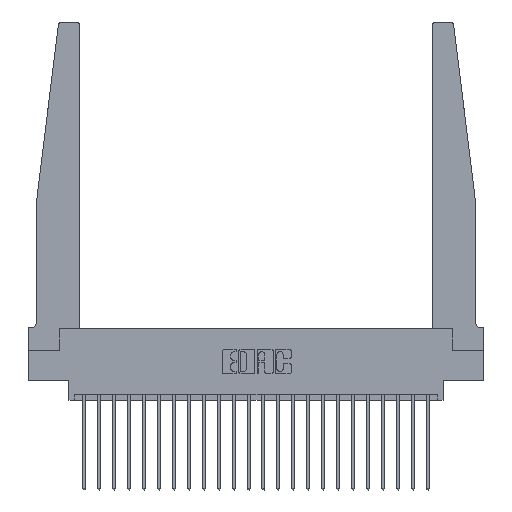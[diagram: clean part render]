
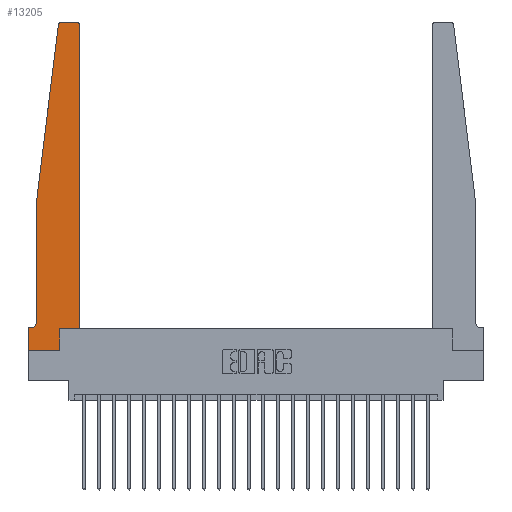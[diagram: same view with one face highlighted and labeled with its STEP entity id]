
A CAD part, top view. The second image highlights one B-rep face of the part: STEP entity #13205.
In plain terms, the highlighted planar face has unit normal (0, 0, 1).
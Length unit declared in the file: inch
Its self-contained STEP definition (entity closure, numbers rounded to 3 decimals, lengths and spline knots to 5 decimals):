
#255 = VECTOR ( 'NONE', #2747, 39.37008 ) ;
#461 = ORIENTED_EDGE ( 'NONE', *, *, #2410, .T. ) ;
#1743 = VECTOR ( 'NONE', #11853, 39.37008 ) ;
#1900 = DIRECTION ( 'NONE',  ( 0., 1., 0. ) ) ;
#1977 = LINE ( 'NONE', #5322, #12302 ) ;
#2410 = EDGE_CURVE ( 'NONE', #17864, #4310, #18258, .T. ) ;
#2473 = DIRECTION ( 'NONE',  ( 0., -1., 0. ) ) ;
#2747 = DIRECTION ( 'NONE',  ( 1., 0., 0. ) ) ;
#2783 = CIRCLE ( 'NONE', #14540, 0.05 ) ;
#3039 = DIRECTION ( 'NONE',  ( 1., 0., 0. ) ) ;
#3114 = LINE ( 'NONE', #15688, #8529 ) ;
#3360 = CARTESIAN_POINT ( 'NONE',  ( 0.425, 0.18, 0.37 ) ) ;
#3427 = CARTESIAN_POINT ( 'NONE',  ( 0.065, 0.2375, 0.37 ) ) ;
#3588 = AXIS2_PLACEMENT_3D ( 'NONE', #8616, #6584, #21063 ) ;
#3815 = VERTEX_POINT ( 'NONE', #21296 ) ;
#4310 = VERTEX_POINT ( 'NONE', #12146 ) ;
#4523 = EDGE_CURVE ( 'NONE', #21504, #8532, #16522, .T. ) ;
#4916 = DIRECTION ( 'NONE',  ( 1., 0., 0. ) ) ;
#4936 = EDGE_CURVE ( 'NONE', #8532, #7044, #9740, .T. ) ;
#5228 = CARTESIAN_POINT ( 'NONE',  ( 0.065, 0.1875, 0.37 ) ) ;
#5322 = CARTESIAN_POINT ( 'NONE',  ( 0.2605, 0.18, 0.37 ) ) ;
#5372 = CARTESIAN_POINT ( 'NONE',  ( 0.25, 2.75, 0.37 ) ) ;
#5847 = FACE_OUTER_BOUND ( 'NONE', #13175, .T. ) ;
#6335 = EDGE_CURVE ( 'NONE', #16356, #3815, #7834, .T. ) ;
#6584 = DIRECTION ( 'NONE',  ( 0., 0., 1. ) ) ;
#6598 = ORIENTED_EDGE ( 'NONE', *, *, #22055, .T. ) ;
#6622 = EDGE_CURVE ( 'NONE', #8867, #16356, #10442, .T. ) ;
#7044 = VERTEX_POINT ( 'NONE', #3427 ) ;
#7380 = CIRCLE ( 'NONE', #16827, 0.03 ) ;
#7487 = ORIENTED_EDGE ( 'NONE', *, *, #20773, .T. ) ;
#7520 = DIRECTION ( 'NONE',  ( 1., 0., 0. ) ) ;
#7834 = LINE ( 'NONE', #22317, #1743 ) ;
#8529 = VECTOR ( 'NONE', #4916, 39.37008 ) ;
#8532 = VERTEX_POINT ( 'NONE', #13611 ) ;
#8574 = CARTESIAN_POINT ( 'NONE',  ( 0.425, 0.18, 0.37 ) ) ;
#8616 = CARTESIAN_POINT ( 'NONE',  ( 0.395, 2.72, 0.37 ) ) ;
#8867 = VERTEX_POINT ( 'NONE', #18564 ) ;
#9093 = CARTESIAN_POINT ( 'NONE',  ( 0.2605, 0.18, 0.37 ) ) ;
#9136 = ORIENTED_EDGE ( 'NONE', *, *, #17896, .T. ) ;
#9294 = CIRCLE ( 'NONE', #3588, 0.03 ) ;
#9361 = VECTOR ( 'NONE', #19211, 39.37008 ) ;
#9436 = DIRECTION ( 'NONE',  ( 0., 0., 1. ) ) ;
#9740 = LINE ( 'NONE', #18731, #20270 ) ;
#10442 = LINE ( 'NONE', #5228, #9361 ) ;
#10521 = CARTESIAN_POINT ( 'NONE',  ( 0.27653, 2.72, 0.37 ) ) ;
#10824 = DIRECTION ( 'NONE',  ( -1., 0., 0. ) ) ;
#11849 = ORIENTED_EDGE ( 'NONE', *, *, #17704, .T. ) ;
#11853 = DIRECTION ( 'NONE',  ( 0., -1., 0. ) ) ;
#12146 = CARTESIAN_POINT ( 'NONE',  ( 0.425, 2.72, 0.37 ) ) ;
#12159 = ORIENTED_EDGE ( 'NONE', *, *, #22575, .T. ) ;
#12302 = VECTOR ( 'NONE', #12549, 39.37008 ) ;
#12487 = LINE ( 'NONE', #5372, #14867 ) ;
#12549 = DIRECTION ( 'NONE',  ( 0., 1., 0. ) ) ;
#12577 = CARTESIAN_POINT ( 'NONE',  ( 0.425, 0.18, 0.37 ) ) ;
#12578 = CARTESIAN_POINT ( 'NONE',  ( 0.27653, 2.75, 0.37 ) ) ;
#13132 = DIRECTION ( 'NONE',  ( -1., 0., 0. ) ) ;
#13175 = EDGE_LOOP ( 'NONE', ( #9136, #6598, #21578, #17922, #7487, #20147, #20325, #12159, #22041, #11849, #461, #21487 ) ) ;
#13205 = ADVANCED_FACE ( 'NONE', ( #5847 ), #20439, .T. ) ;
#13597 = CARTESIAN_POINT ( 'NONE',  ( 0.015, 0.2375, 0.37 ) ) ;
#13611 = CARTESIAN_POINT ( 'NONE',  ( 0.065, 1.25, 0.37 ) ) ;
#14508 = DIRECTION ( 'NONE',  ( -0.122, -0.992, 0. ) ) ;
#14540 = AXIS2_PLACEMENT_3D ( 'NONE', #13597, #20829, #13132 ) ;
#14867 = VECTOR ( 'NONE', #10824, 39.37008 ) ;
#15262 = VECTOR ( 'NONE', #1900, 39.37008 ) ;
#15624 = VERTEX_POINT ( 'NONE', #22748 ) ;
#15688 = CARTESIAN_POINT ( 'NONE',  ( 0., 0., 0.37 ) ) ;
#16356 = VERTEX_POINT ( 'NONE', #18892 ) ;
#16471 = VERTEX_POINT ( 'NONE', #21612 ) ;
#16507 = CARTESIAN_POINT ( 'NONE',  ( 0.24675, 2.72367, 0.37 ) ) ;
#16522 = LINE ( 'NONE', #18185, #16820 ) ;
#16820 = VECTOR ( 'NONE', #14508, 39.37008 ) ;
#16827 = AXIS2_PLACEMENT_3D ( 'NONE', #10521, #19287, #3039 ) ;
#17704 = EDGE_CURVE ( 'NONE', #20975, #17864, #19004, .T. ) ;
#17864 = VERTEX_POINT ( 'NONE', #3360 ) ;
#17896 = EDGE_CURVE ( 'NONE', #15624, #23111, #12487, .T. ) ;
#17922 = ORIENTED_EDGE ( 'NONE', *, *, #4936, .T. ) ;
#18185 = CARTESIAN_POINT ( 'NONE',  ( 0.065, 1.25, 0.37 ) ) ;
#18258 = LINE ( 'NONE', #12577, #15262 ) ;
#18418 = CARTESIAN_POINT ( 'NONE',  ( 0., 0.1875, 0.37 ) ) ;
#18564 = CARTESIAN_POINT ( 'NONE',  ( 0.015, 0.1875, 0.37 ) ) ;
#18731 = CARTESIAN_POINT ( 'NONE',  ( 0.065, 1.25, 0.37 ) ) ;
#18892 = CARTESIAN_POINT ( 'NONE',  ( 0., 0.1875, 0.37 ) ) ;
#19004 = LINE ( 'NONE', #8574, #255 ) ;
#19211 = DIRECTION ( 'NONE',  ( -1., 0., 0. ) ) ;
#19287 = DIRECTION ( 'NONE',  ( 0., 0., 1. ) ) ;
#20147 = ORIENTED_EDGE ( 'NONE', *, *, #6622, .T. ) ;
#20270 = VECTOR ( 'NONE', #2473, 39.37008 ) ;
#20325 = ORIENTED_EDGE ( 'NONE', *, *, #6335, .T. ) ;
#20439 = PLANE ( 'NONE',  #22906 ) ;
#20607 = EDGE_CURVE ( 'NONE', #16471, #20975, #1977, .T. ) ;
#20773 = EDGE_CURVE ( 'NONE', #7044, #8867, #2783, .T. ) ;
#20829 = DIRECTION ( 'NONE',  ( 0., 0., -1. ) ) ;
#20975 = VERTEX_POINT ( 'NONE', #9093 ) ;
#21063 = DIRECTION ( 'NONE',  ( 1., 0., 0. ) ) ;
#21296 = CARTESIAN_POINT ( 'NONE',  ( 0., 0., 0.37 ) ) ;
#21487 = ORIENTED_EDGE ( 'NONE', *, *, #22040, .T. ) ;
#21504 = VERTEX_POINT ( 'NONE', #16507 ) ;
#21578 = ORIENTED_EDGE ( 'NONE', *, *, #4523, .T. ) ;
#21612 = CARTESIAN_POINT ( 'NONE',  ( 0.2605, 0., 0.37 ) ) ;
#22040 = EDGE_CURVE ( 'NONE', #4310, #15624, #9294, .T. ) ;
#22041 = ORIENTED_EDGE ( 'NONE', *, *, #20607, .T. ) ;
#22055 = EDGE_CURVE ( 'NONE', #23111, #21504, #7380, .T. ) ;
#22317 = CARTESIAN_POINT ( 'NONE',  ( 0., 0., 0.37 ) ) ;
#22575 = EDGE_CURVE ( 'NONE', #3815, #16471, #3114, .T. ) ;
#22748 = CARTESIAN_POINT ( 'NONE',  ( 0.395, 2.75, 0.37 ) ) ;
#22906 = AXIS2_PLACEMENT_3D ( 'NONE', #18418, #9436, #7520 ) ;
#23111 = VERTEX_POINT ( 'NONE', #12578 ) ;
